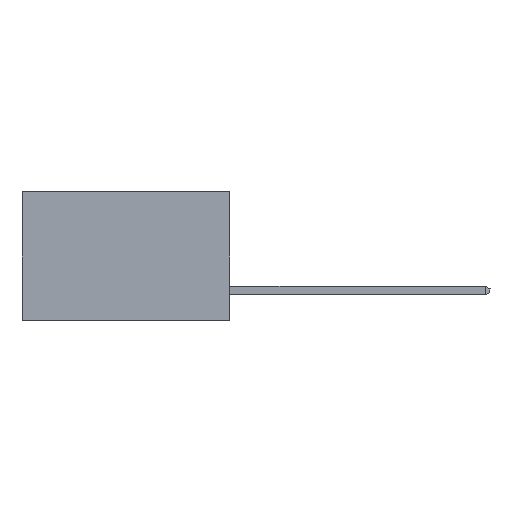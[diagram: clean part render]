
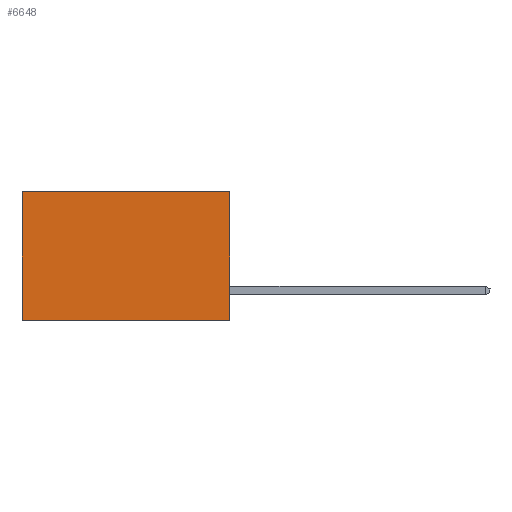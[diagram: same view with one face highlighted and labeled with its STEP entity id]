
A CAD part, left-side view. The second image highlights one B-rep face of the part: STEP entity #6648.
In plain terms, the highlighted planar face has unit normal (-1, 0, 0).
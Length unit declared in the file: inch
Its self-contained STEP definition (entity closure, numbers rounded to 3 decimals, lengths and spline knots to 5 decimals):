
#117 = DIRECTION ( 'NONE',  ( 0., 0., -1. ) ) ;
#1570 = ORIENTED_EDGE ( 'NONE', *, *, #9997, .F. ) ;
#2791 = CARTESIAN_POINT ( 'NONE',  ( 0.2615, 0., -0.37 ) ) ;
#2868 = DIRECTION ( 'NONE',  ( 0., 0., -1. ) ) ;
#4896 = VERTEX_POINT ( 'NONE', #10869 ) ;
#5296 = CARTESIAN_POINT ( 'NONE',  ( 0.2615, 0.6, -0.37 ) ) ;
#5632 = VERTEX_POINT ( 'NONE', #10358 ) ;
#5993 = ORIENTED_EDGE ( 'NONE', *, *, #15189, .T. ) ;
#6004 = EDGE_CURVE ( 'NONE', #15601, #5632, #7728, .T. ) ;
#6388 = VECTOR ( 'NONE', #10374, 39.37008 ) ;
#6648 = ADVANCED_FACE ( 'NONE', ( #13835 ), #12776, .F. ) ;
#6657 = LINE ( 'NONE', #6806, #6388 ) ;
#6806 = CARTESIAN_POINT ( 'NONE',  ( 0.2615, 0., 0. ) ) ;
#7026 = CARTESIAN_POINT ( 'NONE',  ( 0.2615, 0., -0.37 ) ) ;
#7335 = CARTESIAN_POINT ( 'NONE',  ( 0.2615, 0., -0.37 ) ) ;
#7728 = LINE ( 'NONE', #5296, #14643 ) ;
#8071 = ORIENTED_EDGE ( 'NONE', *, *, #8882, .F. ) ;
#8138 = DIRECTION ( 'NONE',  ( 0., 1., 0. ) ) ;
#8217 = AXIS2_PLACEMENT_3D ( 'NONE', #2791, #9200, #2868 ) ;
#8882 = EDGE_CURVE ( 'NONE', #9127, #5632, #11735, .T. ) ;
#9127 = VERTEX_POINT ( 'NONE', #7335 ) ;
#9200 = DIRECTION ( 'NONE',  ( 1., 0., 0. ) ) ;
#9876 = LINE ( 'NONE', #14927, #10264 ) ;
#9971 = VECTOR ( 'NONE', #8138, 39.37008 ) ;
#9997 = EDGE_CURVE ( 'NONE', #4896, #9127, #9876, .T. ) ;
#10264 = VECTOR ( 'NONE', #117, 39.37008 ) ;
#10358 = CARTESIAN_POINT ( 'NONE',  ( 0.2615, 0.6, -0.37 ) ) ;
#10374 = DIRECTION ( 'NONE',  ( 0., 1., 0. ) ) ;
#10869 = CARTESIAN_POINT ( 'NONE',  ( 0.2615, 0., 0. ) ) ;
#11735 = LINE ( 'NONE', #7026, #9971 ) ;
#11752 = EDGE_LOOP ( 'NONE', ( #15228, #8071, #1570, #5993 ) ) ;
#12776 = PLANE ( 'NONE',  #8217 ) ;
#13168 = CARTESIAN_POINT ( 'NONE',  ( 0.2615, 0.6, 0. ) ) ;
#13835 = FACE_OUTER_BOUND ( 'NONE', #11752, .T. ) ;
#14643 = VECTOR ( 'NONE', #15203, 39.37008 ) ;
#14927 = CARTESIAN_POINT ( 'NONE',  ( 0.2615, 0., -0.37 ) ) ;
#15189 = EDGE_CURVE ( 'NONE', #4896, #15601, #6657, .T. ) ;
#15203 = DIRECTION ( 'NONE',  ( 0., 0., -1. ) ) ;
#15228 = ORIENTED_EDGE ( 'NONE', *, *, #6004, .T. ) ;
#15601 = VERTEX_POINT ( 'NONE', #13168 ) ;
